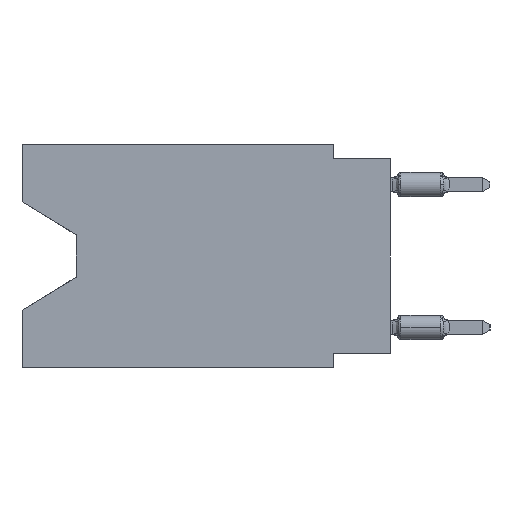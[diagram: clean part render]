
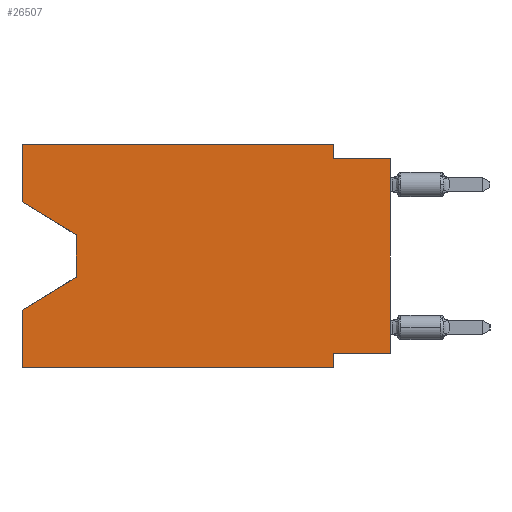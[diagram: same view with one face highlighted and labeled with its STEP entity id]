
A CAD part, left-side view. The second image highlights one B-rep face of the part: STEP entity #26507.
In plain terms, the highlighted planar face has unit normal (-1, 0, 0).
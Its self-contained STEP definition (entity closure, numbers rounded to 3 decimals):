
#882 = CARTESIAN_POINT ( 'NONE',  ( 0., 16.383, -9.906 ) ) ;
#1074 = EDGE_CURVE ( 'NONE', #15115, #27851, #29352, .T. ) ;
#1190 = VERTEX_POINT ( 'NONE', #19733 ) ;
#1471 = VECTOR ( 'NONE', #29360, 1000. ) ;
#1692 = VECTOR ( 'NONE', #15585, 1000. ) ;
#1708 = ORIENTED_EDGE ( 'NONE', *, *, #13857, .F. ) ;
#1718 = ORIENTED_EDGE ( 'NONE', *, *, #23743, .T. ) ;
#1835 = LINE ( 'NONE', #3798, #10200 ) ;
#2994 = LINE ( 'NONE', #21997, #9224 ) ;
#3696 = VECTOR ( 'NONE', #8296, 1000. ) ;
#3798 = CARTESIAN_POINT ( 'NONE',  ( 0., 16.383, 0. ) ) ;
#3815 = LINE ( 'NONE', #10475, #1692 ) ;
#3816 = CARTESIAN_POINT ( 'NONE',  ( 0., 16.383, -2.546 ) ) ;
#4007 = CARTESIAN_POINT ( 'NONE',  ( 0., 16.383, 0. ) ) ;
#4221 = FACE_OUTER_BOUND ( 'NONE', #15422, .T. ) ;
#4851 = CARTESIAN_POINT ( 'NONE',  ( 0., 13.97, -5.893 ) ) ;
#5421 = DIRECTION ( 'NONE',  ( 0., -1., 0. ) ) ;
#5434 = LINE ( 'NONE', #21575, #16581 ) ;
#5983 = ORIENTED_EDGE ( 'NONE', *, *, #21754, .F. ) ;
#6080 = CARTESIAN_POINT ( 'NONE',  ( 0., 16.383, 0. ) ) ;
#6238 = CARTESIAN_POINT ( 'NONE',  ( 0., 16.383, -7.36 ) ) ;
#6294 = DIRECTION ( 'NONE',  ( 0., 0., 1. ) ) ;
#6318 = EDGE_CURVE ( 'NONE', #20479, #12702, #23905, .T. ) ;
#7264 = EDGE_CURVE ( 'NONE', #17868, #13457, #22312, .T. ) ;
#7315 = CARTESIAN_POINT ( 'NONE',  ( 0., 16.383, 0. ) ) ;
#8169 = EDGE_CURVE ( 'NONE', #25330, #17612, #26978, .T. ) ;
#8285 = DIRECTION ( 'NONE',  ( 0., 0., -1. ) ) ;
#8288 = VECTOR ( 'NONE', #25528, 1000. ) ;
#8296 = DIRECTION ( 'NONE',  ( 0., -1., 0. ) ) ;
#8342 = LINE ( 'NONE', #3816, #22103 ) ;
#8609 = DIRECTION ( 'NONE',  ( 1., 0., 0. ) ) ;
#8845 = CARTESIAN_POINT ( 'NONE',  ( 0., 0., 0. ) ) ;
#9224 = VECTOR ( 'NONE', #5421, 1000. ) ;
#9661 = EDGE_CURVE ( 'NONE', #15340, #13457, #2994, .T. ) ;
#10200 = VECTOR ( 'NONE', #22064, 1000. ) ;
#10467 = CARTESIAN_POINT ( 'NONE',  ( 0., 13.97, -4.013 ) ) ;
#10475 = CARTESIAN_POINT ( 'NONE',  ( 0., 0., -9.271 ) ) ;
#11064 = ORIENTED_EDGE ( 'NONE', *, *, #7264, .F. ) ;
#11645 = LINE ( 'NONE', #4851, #22849 ) ;
#11714 = ORIENTED_EDGE ( 'NONE', *, *, #24796, .T. ) ;
#12105 = ORIENTED_EDGE ( 'NONE', *, *, #8169, .F. ) ;
#12301 = DIRECTION ( 'NONE',  ( 0., 0., -1. ) ) ;
#12702 = VERTEX_POINT ( 'NONE', #21591 ) ;
#13320 = DIRECTION ( 'NONE',  ( 0., -0.855, -0.519 ) ) ;
#13348 = ORIENTED_EDGE ( 'NONE', *, *, #28321, .F. ) ;
#13432 = CARTESIAN_POINT ( 'NONE',  ( 0., 2.54, -0.635 ) ) ;
#13457 = VERTEX_POINT ( 'NONE', #16393 ) ;
#13780 = LINE ( 'NONE', #25091, #8288 ) ;
#13851 = CARTESIAN_POINT ( 'NONE',  ( 0., 0., -0.635 ) ) ;
#13857 = EDGE_CURVE ( 'NONE', #27851, #23527, #13780, .T. ) ;
#14048 = VERTEX_POINT ( 'NONE', #6238 ) ;
#14710 = CARTESIAN_POINT ( 'NONE',  ( 0., 2.54, 0. ) ) ;
#15115 = VERTEX_POINT ( 'NONE', #16505 ) ;
#15340 = VERTEX_POINT ( 'NONE', #882 ) ;
#15422 = EDGE_LOOP ( 'NONE', ( #11714, #16021, #1718, #22955, #15995, #11064, #5983, #21352, #12105, #13348, #1708, #27145 ) ) ;
#15585 = DIRECTION ( 'NONE',  ( 0., 1., 0. ) ) ;
#15995 = ORIENTED_EDGE ( 'NONE', *, *, #9661, .T. ) ;
#16021 = ORIENTED_EDGE ( 'NONE', *, *, #6318, .T. ) ;
#16393 = CARTESIAN_POINT ( 'NONE',  ( 0., 2.54, -9.906 ) ) ;
#16505 = CARTESIAN_POINT ( 'NONE',  ( 0., 16.383, -2.546 ) ) ;
#16581 = VECTOR ( 'NONE', #24275, 1000. ) ;
#17169 = CARTESIAN_POINT ( 'NONE',  ( 0., 2.54, -9.271 ) ) ;
#17612 = VERTEX_POINT ( 'NONE', #13851 ) ;
#17868 = VERTEX_POINT ( 'NONE', #17169 ) ;
#17959 = EDGE_CURVE ( 'NONE', #1190, #17612, #18055, .T. ) ;
#18055 = LINE ( 'NONE', #8845, #1471 ) ;
#18834 = EDGE_CURVE ( 'NONE', #15340, #14048, #1835, .T. ) ;
#19655 = VECTOR ( 'NONE', #12301, 1000. ) ;
#19733 = CARTESIAN_POINT ( 'NONE',  ( 0., 0., -9.271 ) ) ;
#20368 = DIRECTION ( 'NONE',  ( 0., 0., -1. ) ) ;
#20479 = VERTEX_POINT ( 'NONE', #10467 ) ;
#21352 = ORIENTED_EDGE ( 'NONE', *, *, #17959, .T. ) ;
#21575 = CARTESIAN_POINT ( 'NONE',  ( 0., 2.54, 0. ) ) ;
#21591 = CARTESIAN_POINT ( 'NONE',  ( 0., 13.97, -5.893 ) ) ;
#21754 = EDGE_CURVE ( 'NONE', #1190, #17868, #3815, .T. ) ;
#21997 = CARTESIAN_POINT ( 'NONE',  ( 0., 16.383, -9.906 ) ) ;
#22064 = DIRECTION ( 'NONE',  ( 0., 0., 1. ) ) ;
#22103 = VECTOR ( 'NONE', #13320, 1000. ) ;
#22312 = LINE ( 'NONE', #24865, #25390 ) ;
#22849 = VECTOR ( 'NONE', #23111, 1000. ) ;
#22955 = ORIENTED_EDGE ( 'NONE', *, *, #18834, .F. ) ;
#23111 = DIRECTION ( 'NONE',  ( 0., 0.855, -0.519 ) ) ;
#23527 = VERTEX_POINT ( 'NONE', #14710 ) ;
#23743 = EDGE_CURVE ( 'NONE', #12702, #14048, #11645, .T. ) ;
#23755 = CARTESIAN_POINT ( 'NONE',  ( 0., 13.97, -4.013 ) ) ;
#23905 = LINE ( 'NONE', #23755, #19655 ) ;
#24275 = DIRECTION ( 'NONE',  ( 0., 0., -1. ) ) ;
#24724 = CARTESIAN_POINT ( 'NONE',  ( 0., 0., -0.635 ) ) ;
#24796 = EDGE_CURVE ( 'NONE', #15115, #20479, #8342, .T. ) ;
#24865 = CARTESIAN_POINT ( 'NONE',  ( 0., 2.54, -9.906 ) ) ;
#24935 = AXIS2_PLACEMENT_3D ( 'NONE', #6080, #8609, #20368 ) ;
#25091 = CARTESIAN_POINT ( 'NONE',  ( 0., 16.383, 0. ) ) ;
#25330 = VERTEX_POINT ( 'NONE', #13432 ) ;
#25390 = VECTOR ( 'NONE', #8285, 1000. ) ;
#25528 = DIRECTION ( 'NONE',  ( 0., -1., 0. ) ) ;
#26507 = ADVANCED_FACE ( 'NONE', ( #4221 ), #26714, .F. ) ;
#26714 = PLANE ( 'NONE',  #24935 ) ;
#26774 = VECTOR ( 'NONE', #6294, 1000. ) ;
#26978 = LINE ( 'NONE', #24724, #3696 ) ;
#27145 = ORIENTED_EDGE ( 'NONE', *, *, #1074, .F. ) ;
#27851 = VERTEX_POINT ( 'NONE', #7315 ) ;
#28321 = EDGE_CURVE ( 'NONE', #23527, #25330, #5434, .T. ) ;
#29352 = LINE ( 'NONE', #4007, #26774 ) ;
#29360 = DIRECTION ( 'NONE',  ( 0., 0., 1. ) ) ;
